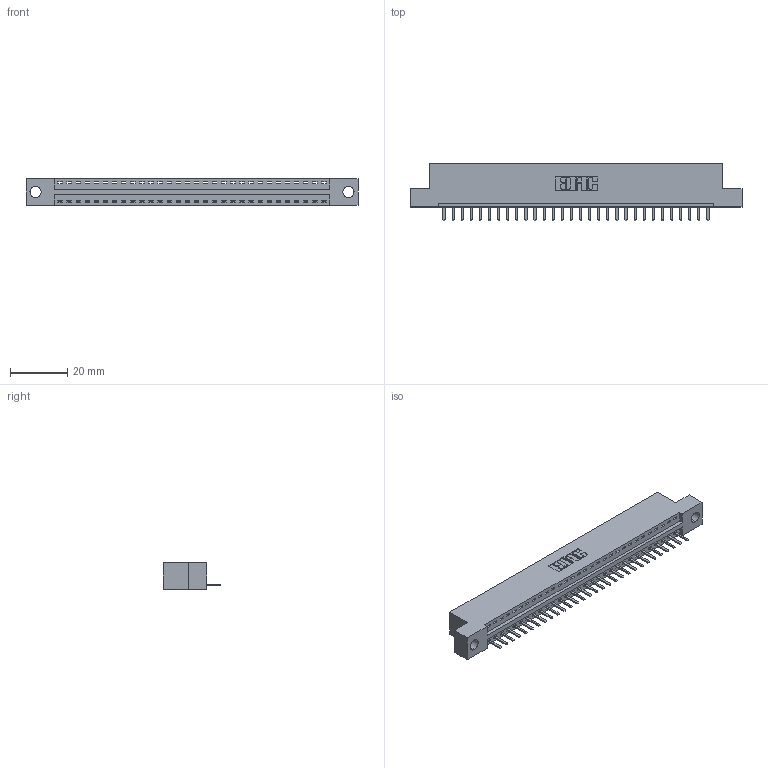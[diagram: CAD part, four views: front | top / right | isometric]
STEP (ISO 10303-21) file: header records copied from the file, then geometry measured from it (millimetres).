
FILE_DESCRIPTION (( 'STEP AP203' ), '1' );
FILE_NAME ('396-030-520-104.STEP', '2018-09-05T05:51:30', ( '' ), ( '' ), 'SwSTEP 2.0', 'SolidWorks 2016', '' );
FILE_SCHEMA (( 'CONFIG_CONTROL_DESIGN' ));
Length unit declared in the file: inch
Products named in the file (3): 346 Part_Flush Mounting Lugs - 0.156 Dia-TH; 345-292-001_345-293-120; 396-030-520-104
Assembly tree (31 placements, depth 2):
  396-030-520-104
    346 Part_Flush Mounting Lugs - 0.156 Dia-TH
    345-292-001_345-293-120  x30
Bounding box: 115.82 x 20.02 x 9.4 mm (x, y, z)
Volume: 10830.1 mm3; surface area: 12923.6 mm2
Topology: 31 solids, 31 shells, 1982 faces, 5849 edges, 3818 vertices
Faces by surface type: plane 1336, cylinder 646
Entity records: 20351 total; most frequent: CARTESIAN_POINT 3510, ORIENTED_EDGE 3462, DIRECTION 3099, EDGE_CURVE 1731, LINE 1475, VECTOR 1475, VERTEX_POINT 1150, AXIS2_PLACEMENT_3D 812
